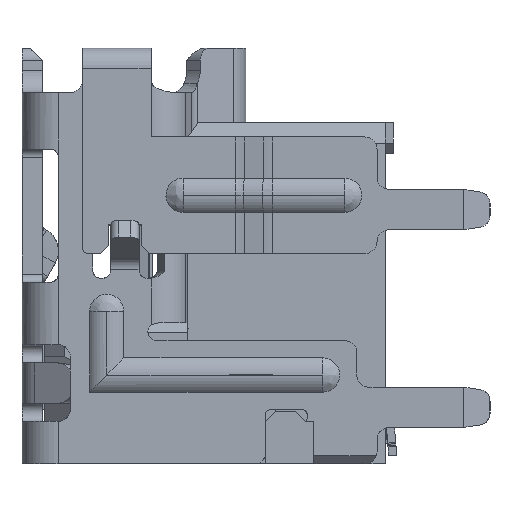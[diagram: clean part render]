
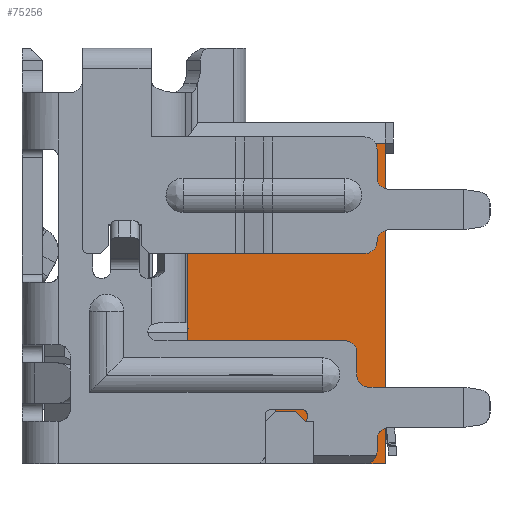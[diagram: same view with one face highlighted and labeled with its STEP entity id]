
A CAD part, left-side view. The second image highlights one B-rep face of the part: STEP entity #75256.
In plain terms, the highlighted planar face has unit normal (-1, 0, 0).
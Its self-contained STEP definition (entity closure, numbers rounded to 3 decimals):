
#11 = CARTESIAN_POINT ( 'NONE',  ( -6.95, -3.575, -4.5 ) ) ;
#215 = VECTOR ( 'NONE', #22734, 1000. ) ;
#997 = ORIENTED_EDGE ( 'NONE', *, *, #66234, .T. ) ;
#2086 = ORIENTED_EDGE ( 'NONE', *, *, #70800, .T. ) ;
#2730 = AXIS2_PLACEMENT_3D ( 'NONE', #16484, #39839, #48444 ) ;
#6080 = EDGE_CURVE ( 'NONE', #16686, #27546, #70881, .T. ) ;
#8572 = ORIENTED_EDGE ( 'NONE', *, *, #89470, .T. ) ;
#8737 = VERTEX_POINT ( 'NONE', #37773 ) ;
#10265 = CARTESIAN_POINT ( 'NONE',  ( -6.95, -3.575, -6.2 ) ) ;
#13669 = VECTOR ( 'NONE', #32244, 1000. ) ;
#15416 = ORIENTED_EDGE ( 'NONE', *, *, #93670, .T. ) ;
#16484 = CARTESIAN_POINT ( 'NONE',  ( -6.95, -3.477, -7.959 ) ) ;
#16686 = VERTEX_POINT ( 'NONE', #40121 ) ;
#20074 = EDGE_LOOP ( 'NONE', ( #997, #78882, #23063, #8572, #2086, #15416, #76785, #70516, #38760, #21393 ) ) ;
#21393 = ORIENTED_EDGE ( 'NONE', *, *, #27253, .T. ) ;
#22734 = DIRECTION ( 'NONE',  ( 0., 0., -1. ) ) ;
#23063 = ORIENTED_EDGE ( 'NONE', *, *, #47950, .T. ) ;
#23182 = CARTESIAN_POINT ( 'NONE',  ( -6.95, -8.475, -7.969 ) ) ;
#26918 = CARTESIAN_POINT ( 'NONE',  ( -6.95, -3.575, -7.959 ) ) ;
#27253 = EDGE_CURVE ( 'NONE', #27546, #39848, #89775, .T. ) ;
#27546 = VERTEX_POINT ( 'NONE', #74931 ) ;
#28472 = VERTEX_POINT ( 'NONE', #70637 ) ;
#29104 = CARTESIAN_POINT ( 'NONE',  ( -6.95, -3.477, -6.5 ) ) ;
#30743 = VERTEX_POINT ( 'NONE', #11 ) ;
#31491 = VERTEX_POINT ( 'NONE', #37687 ) ;
#32244 = DIRECTION ( 'NONE',  ( 0., -0.707, -0.707 ) ) ;
#32735 = CARTESIAN_POINT ( 'NONE',  ( -6.95, -6.25, -6.5 ) ) ;
#34370 = LINE ( 'NONE', #66304, #66956 ) ;
#35465 = DIRECTION ( 'NONE',  ( 0., -1., 0. ) ) ;
#35837 = VECTOR ( 'NONE', #81654, 1000. ) ;
#36695 = VERTEX_POINT ( 'NONE', #80128 ) ;
#37687 = CARTESIAN_POINT ( 'NONE',  ( -6.95, -6.25, -6.5 ) ) ;
#37773 = CARTESIAN_POINT ( 'NONE',  ( -6.95, -6.5, -6.75 ) ) ;
#37978 = LINE ( 'NONE', #83606, #215 ) ;
#38760 = ORIENTED_EDGE ( 'NONE', *, *, #6080, .T. ) ;
#39422 = DIRECTION ( 'NONE',  ( 0., 0., 1. ) ) ;
#39839 = DIRECTION ( 'NONE',  ( -1., 0., 0. ) ) ;
#39848 = VERTEX_POINT ( 'NONE', #100204 ) ;
#40121 = CARTESIAN_POINT ( 'NONE',  ( -6.95, -8.475, -7.8 ) ) ;
#41375 = LINE ( 'NONE', #32735, #13669 ) ;
#42150 = LINE ( 'NONE', #26918, #35837 ) ;
#42582 = CARTESIAN_POINT ( 'NONE',  ( -6.95, -6.5, -7.8 ) ) ;
#45124 = CARTESIAN_POINT ( 'NONE',  ( -6.95, -3.477, 0.15 ) ) ;
#45482 = CARTESIAN_POINT ( 'NONE',  ( -6.95, -3.477, -7.8 ) ) ;
#47950 = EDGE_CURVE ( 'NONE', #83838, #36695, #52223, .T. ) ;
#48444 = DIRECTION ( 'NONE',  ( 0., 0., 1. ) ) ;
#49947 = VECTOR ( 'NONE', #76399, 1000. ) ;
#50224 = DIRECTION ( 'NONE',  ( 0., 0., 1. ) ) ;
#52223 = LINE ( 'NONE', #89737, #88742 ) ;
#54957 = EDGE_CURVE ( 'NONE', #83838, #30743, #63954, .T. ) ;
#55019 = VERTEX_POINT ( 'NONE', #42582 ) ;
#56740 = DIRECTION ( 'NONE',  ( 0., 0., -1. ) ) ;
#63954 = LINE ( 'NONE', #94869, #81318 ) ;
#65005 = VECTOR ( 'NONE', #39422, 1000. ) ;
#66234 = EDGE_CURVE ( 'NONE', #39848, #30743, #42150, .T. ) ;
#66304 = CARTESIAN_POINT ( 'NONE',  ( -6.95, -6.5, -7.959 ) ) ;
#66956 = VECTOR ( 'NONE', #56740, 1000. ) ;
#70516 = ORIENTED_EDGE ( 'NONE', *, *, #77302, .T. ) ;
#70637 = CARTESIAN_POINT ( 'NONE',  ( -6.95, -5.75, -6.5 ) ) ;
#70800 = EDGE_CURVE ( 'NONE', #28472, #31491, #90483, .T. ) ;
#70881 = LINE ( 'NONE', #23182, #65005 ) ;
#74931 = CARTESIAN_POINT ( 'NONE',  ( -6.95, -8.475, 0.15 ) ) ;
#75256 = ADVANCED_FACE ( 'NONE', ( #85966 ), #94085, .T. ) ;
#76399 = DIRECTION ( 'NONE',  ( 0., -1., 0. ) ) ;
#76785 = ORIENTED_EDGE ( 'NONE', *, *, #94314, .T. ) ;
#77302 = EDGE_CURVE ( 'NONE', #55019, #16686, #84511, .T. ) ;
#78882 = ORIENTED_EDGE ( 'NONE', *, *, #54957, .F. ) ;
#80128 = CARTESIAN_POINT ( 'NONE',  ( -6.95, -5.75, -6.2 ) ) ;
#81318 = VECTOR ( 'NONE', #50224, 1000. ) ;
#81654 = DIRECTION ( 'NONE',  ( 0., 0., -1. ) ) ;
#81810 = VECTOR ( 'NONE', #90980, 1000. ) ;
#83473 = VECTOR ( 'NONE', #99383, 1000. ) ;
#83606 = CARTESIAN_POINT ( 'NONE',  ( -6.95, -5.75, -7.959 ) ) ;
#83838 = VERTEX_POINT ( 'NONE', #10265 ) ;
#84511 = LINE ( 'NONE', #45482, #49947 ) ;
#85966 = FACE_OUTER_BOUND ( 'NONE', #20074, .T. ) ;
#88742 = VECTOR ( 'NONE', #35465, 1000. ) ;
#89470 = EDGE_CURVE ( 'NONE', #36695, #28472, #37978, .T. ) ;
#89737 = CARTESIAN_POINT ( 'NONE',  ( -6.95, -3.477, -6.2 ) ) ;
#89775 = LINE ( 'NONE', #45124, #83473 ) ;
#90483 = LINE ( 'NONE', #29104, #81810 ) ;
#90980 = DIRECTION ( 'NONE',  ( 0., -1., 0. ) ) ;
#93670 = EDGE_CURVE ( 'NONE', #31491, #8737, #41375, .T. ) ;
#94085 = PLANE ( 'NONE',  #2730 ) ;
#94314 = EDGE_CURVE ( 'NONE', #8737, #55019, #34370, .T. ) ;
#94869 = CARTESIAN_POINT ( 'NONE',  ( -6.95, -3.575, -4.464 ) ) ;
#99383 = DIRECTION ( 'NONE',  ( 0., 1., 0. ) ) ;
#100204 = CARTESIAN_POINT ( 'NONE',  ( -6.95, -3.575, 0.15 ) ) ;
